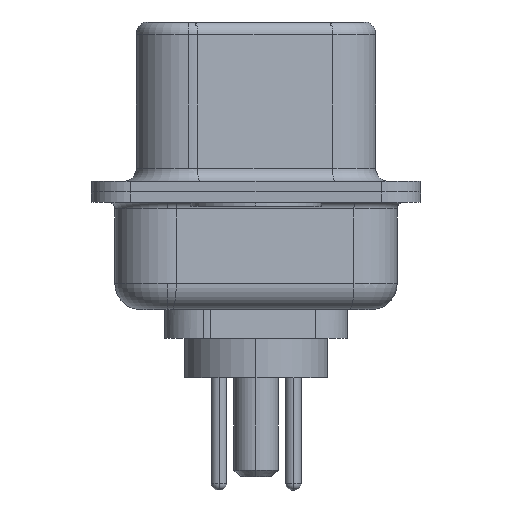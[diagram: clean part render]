
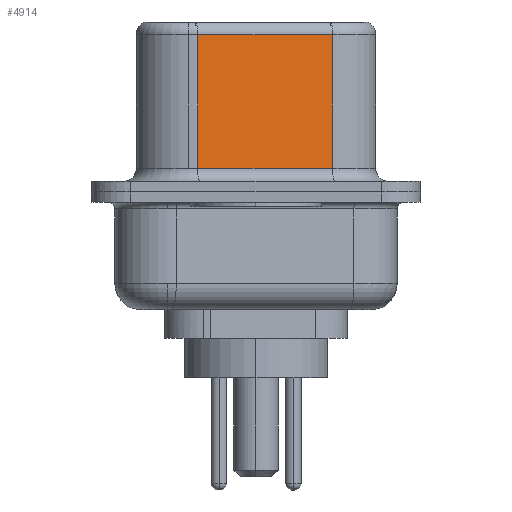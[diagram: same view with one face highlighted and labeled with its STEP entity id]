
A CAD part, left-side view. The second image highlights one B-rep face of the part: STEP entity #4914.
In plain terms, the highlighted planar face has unit normal (-0.985, -0.174, 0).
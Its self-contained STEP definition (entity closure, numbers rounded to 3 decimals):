
#57 = VECTOR ( 'NONE', #13250, 1000. ) ;
#455 = VERTEX_POINT ( 'NONE', #17858 ) ;
#512 = LINE ( 'NONE', #2633, #57 ) ;
#784 = ORIENTED_EDGE ( 'NONE', *, *, #7678, .T. ) ;
#874 = LINE ( 'NONE', #11882, #8372 ) ;
#1207 = VECTOR ( 'NONE', #16781, 1000. ) ;
#1304 = DIRECTION ( 'NONE',  ( 0., 0., -1. ) ) ;
#2633 = CARTESIAN_POINT ( 'NONE',  ( 4.58, -2.927, 0.9 ) ) ;
#2738 = CARTESIAN_POINT ( 'NONE',  ( 3.67, 2.233, 0.9 ) ) ;
#3009 = DIRECTION ( 'NONE',  ( -0.174, 0.985, 0. ) ) ;
#3378 = CARTESIAN_POINT ( 'NONE',  ( 4.58, -2.927, 6.52 ) ) ;
#3763 = LINE ( 'NONE', #17874, #18966 ) ;
#4741 = VERTEX_POINT ( 'NONE', #2738 ) ;
#4914 = ADVANCED_FACE ( 'NONE', ( #13748 ), #16103, .F. ) ;
#5047 = EDGE_CURVE ( 'NONE', #455, #4741, #3763, .T. ) ;
#6065 = EDGE_CURVE ( 'NONE', #15403, #19546, #16836, .T. ) ;
#7678 = EDGE_CURVE ( 'NONE', #15403, #455, #874, .T. ) ;
#8372 = VECTOR ( 'NONE', #3009, 1000. ) ;
#9023 = ORIENTED_EDGE ( 'NONE', *, *, #5047, .T. ) ;
#10304 = ORIENTED_EDGE ( 'NONE', *, *, #6065, .F. ) ;
#10362 = CARTESIAN_POINT ( 'NONE',  ( 4.58, -2.927, 0.9 ) ) ;
#10973 = DIRECTION ( 'NONE',  ( -0.174, 0.985, 0. ) ) ;
#11882 = CARTESIAN_POINT ( 'NONE',  ( 4.58, -2.927, 6.02 ) ) ;
#13250 = DIRECTION ( 'NONE',  ( 0.174, -0.985, 0. ) ) ;
#13409 = ORIENTED_EDGE ( 'NONE', *, *, #19450, .T. ) ;
#13748 = FACE_OUTER_BOUND ( 'NONE', #14553, .T. ) ;
#14553 = EDGE_LOOP ( 'NONE', ( #10304, #784, #9023, #13409 ) ) ;
#14901 = DIRECTION ( 'NONE',  ( 0.985, 0.174, 0. ) ) ;
#15280 = CARTESIAN_POINT ( 'NONE',  ( 4.58, -2.927, 6.52 ) ) ;
#15403 = VERTEX_POINT ( 'NONE', #17565 ) ;
#16103 = PLANE ( 'NONE',  #18818 ) ;
#16781 = DIRECTION ( 'NONE',  ( 0., 0., -1. ) ) ;
#16836 = LINE ( 'NONE', #15280, #1207 ) ;
#17565 = CARTESIAN_POINT ( 'NONE',  ( 4.58, -2.927, 6.02 ) ) ;
#17858 = CARTESIAN_POINT ( 'NONE',  ( 3.67, 2.233, 6.02 ) ) ;
#17874 = CARTESIAN_POINT ( 'NONE',  ( 3.67, 2.233, 6.52 ) ) ;
#18818 = AXIS2_PLACEMENT_3D ( 'NONE', #3378, #14901, #10973 ) ;
#18966 = VECTOR ( 'NONE', #1304, 1000. ) ;
#19450 = EDGE_CURVE ( 'NONE', #4741, #19546, #512, .T. ) ;
#19546 = VERTEX_POINT ( 'NONE', #10362 ) ;
